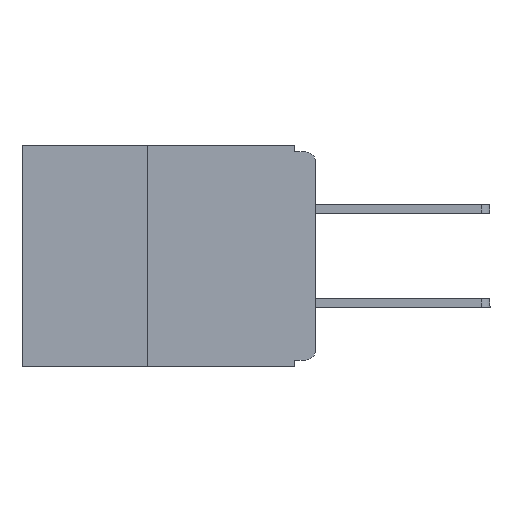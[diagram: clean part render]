
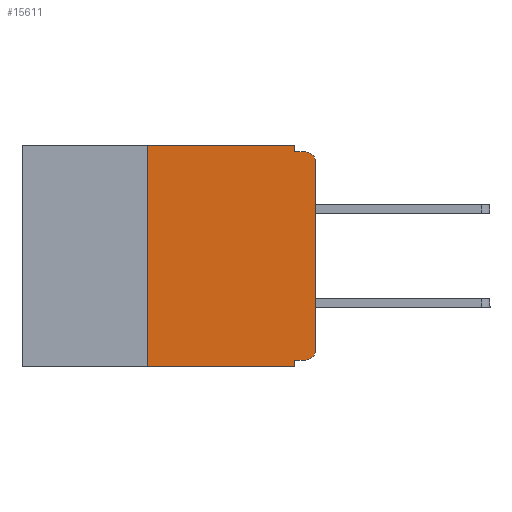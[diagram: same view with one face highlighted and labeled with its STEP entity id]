
A CAD part, left-side view. The second image highlights one B-rep face of the part: STEP entity #15611.
In plain terms, the highlighted planar face has unit normal (-1, 0, 0).
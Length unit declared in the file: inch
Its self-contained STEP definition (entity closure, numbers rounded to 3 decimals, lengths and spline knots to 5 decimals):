
#195 = CARTESIAN_POINT ( 'NONE',  ( 0., 0.015, -0.01 ) ) ;
#199 = EDGE_LOOP ( 'NONE', ( #11464, #1737, #3664, #8487, #11109, #14859, #20964, #2601, #2577, #2887 ) ) ;
#370 = EDGE_CURVE ( 'NONE', #12213, #8527, #7542, .T. ) ;
#713 = VERTEX_POINT ( 'NONE', #2820 ) ;
#1123 = DIRECTION ( 'NONE',  ( 0., 1., 0. ) ) ;
#1143 = CARTESIAN_POINT ( 'NONE',  ( 0., 0., -0.01 ) ) ;
#1400 = CARTESIAN_POINT ( 'NONE',  ( 0., 0.25, -0.33 ) ) ;
#1483 = CARTESIAN_POINT ( 'NONE',  ( 0., 0.25, 0. ) ) ;
#1658 = CARTESIAN_POINT ( 'NONE',  ( 0., 0.015, -0.025 ) ) ;
#1737 = ORIENTED_EDGE ( 'NONE', *, *, #14193, .T. ) ;
#1851 = CARTESIAN_POINT ( 'NONE',  ( 0., 0.031, 0. ) ) ;
#2079 = CARTESIAN_POINT ( 'NONE',  ( 0., 0.015, -0.305 ) ) ;
#2577 = ORIENTED_EDGE ( 'NONE', *, *, #14611, .F. ) ;
#2601 = ORIENTED_EDGE ( 'NONE', *, *, #370, .F. ) ;
#2610 = LINE ( 'NONE', #3282, #20023 ) ;
#2820 = CARTESIAN_POINT ( 'NONE',  ( 0., 0., -0.305 ) ) ;
#2887 = ORIENTED_EDGE ( 'NONE', *, *, #21697, .T. ) ;
#3157 = CARTESIAN_POINT ( 'NONE',  ( 0., 0., -0.025 ) ) ;
#3282 = CARTESIAN_POINT ( 'NONE',  ( 0., 0.25, -0.33 ) ) ;
#3395 = DIRECTION ( 'NONE',  ( 0., 0., -1. ) ) ;
#3664 = ORIENTED_EDGE ( 'NONE', *, *, #16524, .F. ) ;
#3772 = DIRECTION ( 'NONE',  ( 0., 0., -1. ) ) ;
#4299 = EDGE_CURVE ( 'NONE', #713, #12926, #15363, .T. ) ;
#4930 = CARTESIAN_POINT ( 'NONE',  ( 0., 0.437, 0. ) ) ;
#5288 = CARTESIAN_POINT ( 'NONE',  ( 0., 0.031, -0.33 ) ) ;
#6655 = DIRECTION ( 'NONE',  ( 0., -1., 0. ) ) ;
#7110 = DIRECTION ( 'NONE',  ( 0., 0., -1. ) ) ;
#7241 = VERTEX_POINT ( 'NONE', #17506 ) ;
#7542 = LINE ( 'NONE', #5288, #16160 ) ;
#7710 = DIRECTION ( 'NONE',  ( 0., 0., -1. ) ) ;
#8183 = LINE ( 'NONE', #9719, #12307 ) ;
#8455 = DIRECTION ( 'NONE',  ( 0., 0., 1. ) ) ;
#8487 = ORIENTED_EDGE ( 'NONE', *, *, #10306, .F. ) ;
#8527 = VERTEX_POINT ( 'NONE', #13914 ) ;
#9039 = VECTOR ( 'NONE', #6655, 39.37008 ) ;
#9208 = VECTOR ( 'NONE', #18774, 39.37008 ) ;
#9567 = LINE ( 'NONE', #1143, #13648 ) ;
#9597 = CIRCLE ( 'NONE', #15753, 0.015 ) ;
#9719 = CARTESIAN_POINT ( 'NONE',  ( 0., 0., -0.32 ) ) ;
#10025 = VERTEX_POINT ( 'NONE', #19811 ) ;
#10300 = VECTOR ( 'NONE', #16672, 39.37008 ) ;
#10306 = EDGE_CURVE ( 'NONE', #20932, #7241, #13830, .T. ) ;
#11109 = ORIENTED_EDGE ( 'NONE', *, *, #14165, .F. ) ;
#11409 = AXIS2_PLACEMENT_3D ( 'NONE', #15746, #17348, #7110 ) ;
#11464 = ORIENTED_EDGE ( 'NONE', *, *, #4299, .T. ) ;
#12213 = VERTEX_POINT ( 'NONE', #15714 ) ;
#12307 = VECTOR ( 'NONE', #1123, 39.37008 ) ;
#12602 = VERTEX_POINT ( 'NONE', #1400 ) ;
#12926 = VERTEX_POINT ( 'NONE', #3157 ) ;
#13103 = VERTEX_POINT ( 'NONE', #195 ) ;
#13517 = EDGE_CURVE ( 'NONE', #12602, #17303, #2610, .T. ) ;
#13648 = VECTOR ( 'NONE', #14926, 39.37008 ) ;
#13755 = DIRECTION ( 'NONE',  ( -1., 0., 0. ) ) ;
#13830 = LINE ( 'NONE', #1851, #9208 ) ;
#13914 = CARTESIAN_POINT ( 'NONE',  ( 0., 0.031, -0.33 ) ) ;
#14015 = VECTOR ( 'NONE', #15161, 39.37008 ) ;
#14064 = PLANE ( 'NONE',  #11409 ) ;
#14157 = DIRECTION ( 'NONE',  ( -1., 0., 0. ) ) ;
#14165 = EDGE_CURVE ( 'NONE', #17303, #20932, #18024, .T. ) ;
#14193 = EDGE_CURVE ( 'NONE', #12926, #13103, #9597, .T. ) ;
#14566 = CARTESIAN_POINT ( 'NONE',  ( 0., 0.031, 0. ) ) ;
#14611 = EDGE_CURVE ( 'NONE', #10025, #12213, #8183, .T. ) ;
#14859 = ORIENTED_EDGE ( 'NONE', *, *, #13517, .F. ) ;
#14926 = DIRECTION ( 'NONE',  ( 0., -1., 0. ) ) ;
#15066 = LINE ( 'NONE', #18358, #14015 ) ;
#15161 = DIRECTION ( 'NONE',  ( 0., -1., 0. ) ) ;
#15363 = LINE ( 'NONE', #16802, #10300 ) ;
#15611 = ADVANCED_FACE ( 'NONE', ( #15690 ), #14064, .F. ) ;
#15690 = FACE_OUTER_BOUND ( 'NONE', #199, .T. ) ;
#15714 = CARTESIAN_POINT ( 'NONE',  ( 0., 0.031, -0.32 ) ) ;
#15746 = CARTESIAN_POINT ( 'NONE',  ( 0., 0.437, 0. ) ) ;
#15753 = AXIS2_PLACEMENT_3D ( 'NONE', #1658, #13755, #3395 ) ;
#16160 = VECTOR ( 'NONE', #7710, 39.37008 ) ;
#16524 = EDGE_CURVE ( 'NONE', #7241, #13103, #9567, .T. ) ;
#16539 = CIRCLE ( 'NONE', #21066, 0.015 ) ;
#16672 = DIRECTION ( 'NONE',  ( 0., 0., 1. ) ) ;
#16802 = CARTESIAN_POINT ( 'NONE',  ( 0., 0., 0. ) ) ;
#17303 = VERTEX_POINT ( 'NONE', #1483 ) ;
#17348 = DIRECTION ( 'NONE',  ( 1., 0., 0. ) ) ;
#17506 = CARTESIAN_POINT ( 'NONE',  ( 0., 0.031, -0.01 ) ) ;
#18024 = LINE ( 'NONE', #4930, #9039 ) ;
#18358 = CARTESIAN_POINT ( 'NONE',  ( 0., 0.437, -0.33 ) ) ;
#18774 = DIRECTION ( 'NONE',  ( 0., 0., -1. ) ) ;
#19811 = CARTESIAN_POINT ( 'NONE',  ( 0., 0.015, -0.32 ) ) ;
#20023 = VECTOR ( 'NONE', #8455, 39.37008 ) ;
#20573 = EDGE_CURVE ( 'NONE', #12602, #8527, #15066, .T. ) ;
#20932 = VERTEX_POINT ( 'NONE', #14566 ) ;
#20964 = ORIENTED_EDGE ( 'NONE', *, *, #20573, .T. ) ;
#21066 = AXIS2_PLACEMENT_3D ( 'NONE', #2079, #14157, #3772 ) ;
#21697 = EDGE_CURVE ( 'NONE', #10025, #713, #16539, .T. ) ;
